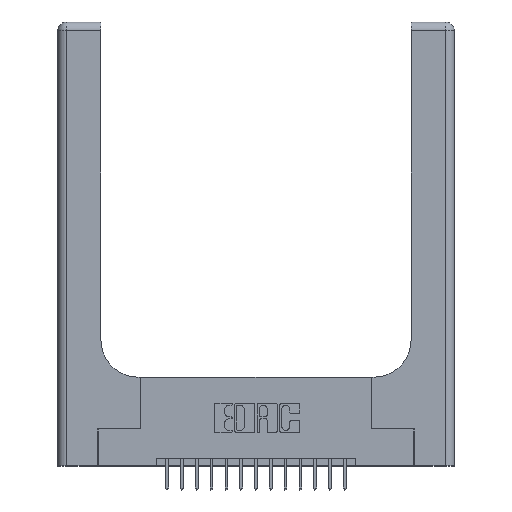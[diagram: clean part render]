
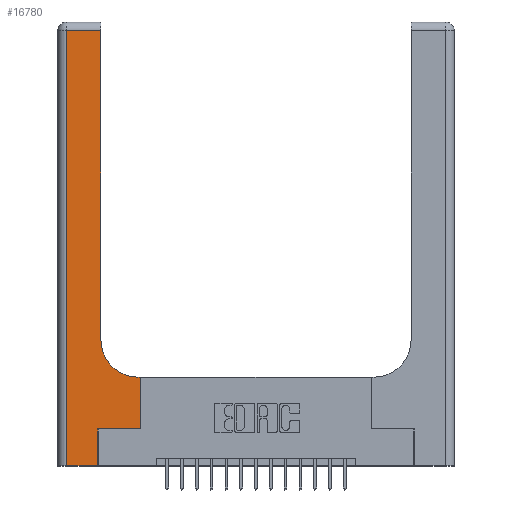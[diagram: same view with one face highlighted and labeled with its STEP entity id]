
A CAD part, top view. The second image highlights one B-rep face of the part: STEP entity #16780.
In plain terms, the highlighted planar face has unit normal (0, 0, 1).
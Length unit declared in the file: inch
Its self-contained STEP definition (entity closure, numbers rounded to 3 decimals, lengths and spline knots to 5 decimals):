
#161 = EDGE_CURVE ( 'NONE', #7240, #14917, #11860, .T. ) ;
#233 = VECTOR ( 'NONE', #18847, 39.37008 ) ;
#350 = VECTOR ( 'NONE', #15846, 39.37008 ) ;
#814 = LINE ( 'NONE', #14329, #350 ) ;
#861 = CARTESIAN_POINT ( 'NONE',  ( 0.269, 0., 0.37 ) ) ;
#1030 = EDGE_CURVE ( 'NONE', #16239, #7240, #6518, .T. ) ;
#1366 = DIRECTION ( 'NONE',  ( 0., -1., 0. ) ) ;
#2018 = CARTESIAN_POINT ( 'NONE',  ( 0.2915, 2.94, 0.37 ) ) ;
#2336 = VECTOR ( 'NONE', #2629, 39.37008 ) ;
#2502 = CARTESIAN_POINT ( 'NONE',  ( 0.269, 0.25, 0.37 ) ) ;
#2524 = EDGE_CURVE ( 'NONE', #17821, #7742, #6222, .T. ) ;
#2629 = DIRECTION ( 'NONE',  ( 1., 0., 0. ) ) ;
#2714 = EDGE_CURVE ( 'NONE', #14917, #7744, #3226, .T. ) ;
#2996 = CARTESIAN_POINT ( 'NONE',  ( 0.06, 3., 0.37 ) ) ;
#3031 = LINE ( 'NONE', #5447, #233 ) ;
#3206 = DIRECTION ( 'NONE',  ( -1., 0., 0. ) ) ;
#3226 = LINE ( 'NONE', #15301, #19138 ) ;
#3334 = DIRECTION ( 'NONE',  ( 0., 0., -1. ) ) ;
#3844 = LINE ( 'NONE', #2996, #6145 ) ;
#3994 = DIRECTION ( 'NONE',  ( 1., 0., 0. ) ) ;
#4086 = CARTESIAN_POINT ( 'NONE',  ( 0.5415, 0.6, 0.37 ) ) ;
#4810 = EDGE_CURVE ( 'NONE', #10527, #17821, #3844, .T. ) ;
#5447 = CARTESIAN_POINT ( 'NONE',  ( 0.2915, 3., 0.37 ) ) ;
#5640 = LINE ( 'NONE', #861, #13124 ) ;
#6082 = ORIENTED_EDGE ( 'NONE', *, *, #18825, .T. ) ;
#6145 = VECTOR ( 'NONE', #1366, 39.37008 ) ;
#6222 = LINE ( 'NONE', #14255, #10907 ) ;
#6467 = AXIS2_PLACEMENT_3D ( 'NONE', #9299, #10911, #10851 ) ;
#6518 = LINE ( 'NONE', #2502, #2336 ) ;
#7183 = VECTOR ( 'NONE', #10377, 39.37008 ) ;
#7240 = VERTEX_POINT ( 'NONE', #11112 ) ;
#7742 = VERTEX_POINT ( 'NONE', #14088 ) ;
#7744 = VERTEX_POINT ( 'NONE', #4086 ) ;
#8068 = CARTESIAN_POINT ( 'NONE',  ( 0.2915, 0.85, 0.37 ) ) ;
#8380 = EDGE_CURVE ( 'NONE', #9247, #10500, #3031, .T. ) ;
#8627 = ORIENTED_EDGE ( 'NONE', *, *, #1030, .T. ) ;
#8668 = CARTESIAN_POINT ( 'NONE',  ( 0.06, 0., 0.37 ) ) ;
#8689 = ORIENTED_EDGE ( 'NONE', *, *, #15696, .T. ) ;
#9198 = CARTESIAN_POINT ( 'NONE',  ( 0., 3., 0.37 ) ) ;
#9247 = VERTEX_POINT ( 'NONE', #8068 ) ;
#9299 = CARTESIAN_POINT ( 'NONE',  ( 0.5415, 0.85, 0.37 ) ) ;
#9330 = CIRCLE ( 'NONE', #6467, 0.25 ) ;
#9914 = ORIENTED_EDGE ( 'NONE', *, *, #8380, .T. ) ;
#10186 = CARTESIAN_POINT ( 'NONE',  ( 0.5585, 0.6, 0.37 ) ) ;
#10377 = DIRECTION ( 'NONE',  ( 0., 1., 0. ) ) ;
#10500 = VERTEX_POINT ( 'NONE', #2018 ) ;
#10527 = VERTEX_POINT ( 'NONE', #10998 ) ;
#10565 = ORIENTED_EDGE ( 'NONE', *, *, #4810, .T. ) ;
#10851 = DIRECTION ( 'NONE',  ( 1., 0., 0. ) ) ;
#10907 = VECTOR ( 'NONE', #3994, 39.37008 ) ;
#10911 = DIRECTION ( 'NONE',  ( 0., 0., -1. ) ) ;
#10998 = CARTESIAN_POINT ( 'NONE',  ( 0.06, 2.94, 0.37 ) ) ;
#11112 = CARTESIAN_POINT ( 'NONE',  ( 0.5585, 0.25, 0.37 ) ) ;
#11832 = ORIENTED_EDGE ( 'NONE', *, *, #2524, .T. ) ;
#11860 = LINE ( 'NONE', #13328, #7183 ) ;
#12138 = CARTESIAN_POINT ( 'NONE',  ( 0.269, 0.25, 0.37 ) ) ;
#12957 = ORIENTED_EDGE ( 'NONE', *, *, #19381, .T. ) ;
#13124 = VECTOR ( 'NONE', #14501, 39.37008 ) ;
#13328 = CARTESIAN_POINT ( 'NONE',  ( 0.5585, 0.25, 0.37 ) ) ;
#13471 = FACE_OUTER_BOUND ( 'NONE', #17855, .T. ) ;
#13756 = PLANE ( 'NONE',  #16435 ) ;
#13834 = DIRECTION ( 'NONE',  ( -1., 0., 0. ) ) ;
#14088 = CARTESIAN_POINT ( 'NONE',  ( 0.269, 0., 0.37 ) ) ;
#14255 = CARTESIAN_POINT ( 'NONE',  ( 0., 0., 0.37 ) ) ;
#14329 = CARTESIAN_POINT ( 'NONE',  ( 0., 2.94, 0.37 ) ) ;
#14501 = DIRECTION ( 'NONE',  ( 0., 1., 0. ) ) ;
#14917 = VERTEX_POINT ( 'NONE', #10186 ) ;
#15301 = CARTESIAN_POINT ( 'NONE',  ( 0.2915, 0.6, 0.37 ) ) ;
#15696 = EDGE_CURVE ( 'NONE', #7744, #9247, #9330, .T. ) ;
#15846 = DIRECTION ( 'NONE',  ( -1., 0., 0. ) ) ;
#16239 = VERTEX_POINT ( 'NONE', #12138 ) ;
#16435 = AXIS2_PLACEMENT_3D ( 'NONE', #9198, #3334, #13834 ) ;
#16780 = ADVANCED_FACE ( 'NONE', ( #13471 ), #13756, .F. ) ;
#17085 = ORIENTED_EDGE ( 'NONE', *, *, #2714, .T. ) ;
#17821 = VERTEX_POINT ( 'NONE', #8668 ) ;
#17855 = EDGE_LOOP ( 'NONE', ( #9914, #6082, #10565, #11832, #12957, #8627, #18594, #17085, #8689 ) ) ;
#18594 = ORIENTED_EDGE ( 'NONE', *, *, #161, .T. ) ;
#18825 = EDGE_CURVE ( 'NONE', #10500, #10527, #814, .T. ) ;
#18847 = DIRECTION ( 'NONE',  ( 0., 1., 0. ) ) ;
#19138 = VECTOR ( 'NONE', #3206, 39.37008 ) ;
#19381 = EDGE_CURVE ( 'NONE', #7742, #16239, #5640, .T. ) ;
